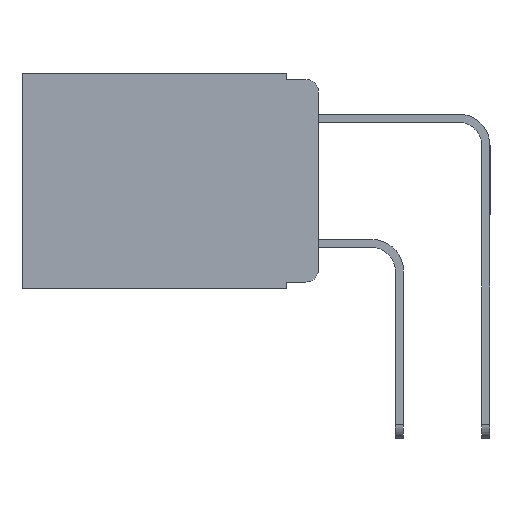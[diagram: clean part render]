
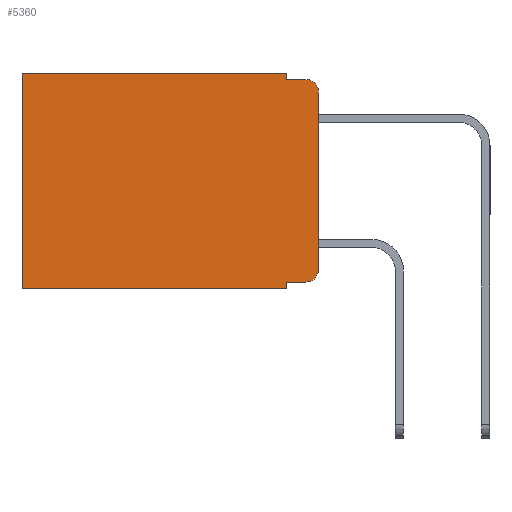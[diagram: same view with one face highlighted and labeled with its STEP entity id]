
A CAD part, left-side view. The second image highlights one B-rep face of the part: STEP entity #5360.
In plain terms, the highlighted planar face has unit normal (-1, 0, 0).
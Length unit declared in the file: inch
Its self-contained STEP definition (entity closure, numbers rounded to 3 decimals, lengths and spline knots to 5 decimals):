
#64 = VERTEX_POINT ( 'NONE', #9106 ) ;
#231 = EDGE_LOOP ( 'NONE', ( #799, #5601, #1090, #2613, #10460, #2832, #511, #421, #3322, #2909 ) ) ;
#248 = EDGE_CURVE ( 'NONE', #4413, #12292, #5980, .T. ) ;
#421 = ORIENTED_EDGE ( 'NONE', *, *, #8925, .F. ) ;
#511 = ORIENTED_EDGE ( 'NONE', *, *, #3131, .F. ) ;
#660 = CARTESIAN_POINT ( 'NONE',  ( 0.298, 0.473, 0. ) ) ;
#770 = CARTESIAN_POINT ( 'NONE',  ( 0.298, 0.051, -0.333 ) ) ;
#799 = ORIENTED_EDGE ( 'NONE', *, *, #2917, .F. ) ;
#839 = EDGE_CURVE ( 'NONE', #64, #4199, #1407, .T. ) ;
#1090 = ORIENTED_EDGE ( 'NONE', *, *, #248, .F. ) ;
#1407 = LINE ( 'NONE', #8912, #4259 ) ;
#1608 = EDGE_CURVE ( 'NONE', #7378, #12292, #6070, .T. ) ;
#1826 = VECTOR ( 'NONE', #3540, 39.37008 ) ;
#1847 = CARTESIAN_POINT ( 'NONE',  ( 0.298, 0.02, -0.313 ) ) ;
#2059 = LINE ( 'NONE', #660, #9380 ) ;
#2218 = DIRECTION ( 'NONE',  ( 0., 0., -1. ) ) ;
#2267 = CIRCLE ( 'NONE', #11400, 0.02 ) ;
#2272 = LINE ( 'NONE', #7502, #11727 ) ;
#2394 = CARTESIAN_POINT ( 'NONE',  ( 0.298, 0.473, -0.343 ) ) ;
#2399 = VECTOR ( 'NONE', #8474, 39.37008 ) ;
#2431 = LINE ( 'NONE', #2488, #1826 ) ;
#2488 = CARTESIAN_POINT ( 'NONE',  ( 0.298, 0., 0. ) ) ;
#2562 = CARTESIAN_POINT ( 'NONE',  ( 0.298, 0.02, -0.333 ) ) ;
#2613 = ORIENTED_EDGE ( 'NONE', *, *, #11981, .F. ) ;
#2786 = VERTEX_POINT ( 'NONE', #2562 ) ;
#2829 = DIRECTION ( 'NONE',  ( 0., 0., -1. ) ) ;
#2832 = ORIENTED_EDGE ( 'NONE', *, *, #10750, .T. ) ;
#2909 = ORIENTED_EDGE ( 'NONE', *, *, #7652, .T. ) ;
#2917 = EDGE_CURVE ( 'NONE', #7378, #9692, #2431, .T. ) ;
#3131 = EDGE_CURVE ( 'NONE', #12172, #10574, #2272, .T. ) ;
#3322 = ORIENTED_EDGE ( 'NONE', *, *, #8294, .T. ) ;
#3540 = DIRECTION ( 'NONE',  ( 0., 0., -1. ) ) ;
#3930 = CARTESIAN_POINT ( 'NONE',  ( 0.298, 0.051, -0.343 ) ) ;
#3992 = CARTESIAN_POINT ( 'NONE',  ( 0.298, 0.473, 0. ) ) ;
#4199 = VERTEX_POINT ( 'NONE', #3992 ) ;
#4259 = VECTOR ( 'NONE', #11810, 39.37008 ) ;
#4413 = VERTEX_POINT ( 'NONE', #5034 ) ;
#5034 = CARTESIAN_POINT ( 'NONE',  ( 0.298, 0.051, -0.01 ) ) ;
#5148 = VECTOR ( 'NONE', #5553, 39.37008 ) ;
#5175 = DIRECTION ( 'NONE',  ( 1., 0., 0. ) ) ;
#5280 = PLANE ( 'NONE',  #8699 ) ;
#5284 = VERTEX_POINT ( 'NONE', #8490 ) ;
#5310 = CARTESIAN_POINT ( 'NONE',  ( 0.298, 0.051, 0. ) ) ;
#5360 = ADVANCED_FACE ( 'NONE', ( #11406 ), #5280, .F. ) ;
#5553 = DIRECTION ( 'NONE',  ( 0., 0., -1. ) ) ;
#5601 = ORIENTED_EDGE ( 'NONE', *, *, #1608, .T. ) ;
#5980 = LINE ( 'NONE', #10342, #9808 ) ;
#6070 = CIRCLE ( 'NONE', #11501, 0.02 ) ;
#6178 = CARTESIAN_POINT ( 'NONE',  ( 0.298, 0., 0. ) ) ;
#7170 = CARTESIAN_POINT ( 'NONE',  ( 0.298, 0., -0.03 ) ) ;
#7378 = VERTEX_POINT ( 'NONE', #7170 ) ;
#7502 = CARTESIAN_POINT ( 'NONE',  ( 0.298, 0., -0.343 ) ) ;
#7509 = LINE ( 'NONE', #770, #2399 ) ;
#7652 = EDGE_CURVE ( 'NONE', #2786, #9692, #2267, .T. ) ;
#7951 = LINE ( 'NONE', #5310, #10117 ) ;
#8294 = EDGE_CURVE ( 'NONE', #5284, #2786, #7509, .T. ) ;
#8474 = DIRECTION ( 'NONE',  ( 0., -1., 0. ) ) ;
#8490 = CARTESIAN_POINT ( 'NONE',  ( 0.298, 0.051, -0.333 ) ) ;
#8573 = DIRECTION ( 'NONE',  ( -1., 0., 0. ) ) ;
#8640 = LINE ( 'NONE', #11189, #5148 ) ;
#8699 = AXIS2_PLACEMENT_3D ( 'NONE', #6178, #5175, #2218 ) ;
#8912 = CARTESIAN_POINT ( 'NONE',  ( 0.298, 0., 0. ) ) ;
#8925 = EDGE_CURVE ( 'NONE', #5284, #12172, #7951, .T. ) ;
#8933 = DIRECTION ( 'NONE',  ( 0., 1., 0. ) ) ;
#8987 = DIRECTION ( 'NONE',  ( 0., -1., 0. ) ) ;
#9106 = CARTESIAN_POINT ( 'NONE',  ( 0.298, 0.051, 0. ) ) ;
#9135 = DIRECTION ( 'NONE',  ( 0., 0., -1. ) ) ;
#9189 = CARTESIAN_POINT ( 'NONE',  ( 0.298, 0.02, -0.03 ) ) ;
#9210 = DIRECTION ( 'NONE',  ( -1., 0., 0. ) ) ;
#9380 = VECTOR ( 'NONE', #10197, 39.37008 ) ;
#9692 = VERTEX_POINT ( 'NONE', #11281 ) ;
#9808 = VECTOR ( 'NONE', #8987, 39.37008 ) ;
#10117 = VECTOR ( 'NONE', #10971, 39.37008 ) ;
#10197 = DIRECTION ( 'NONE',  ( 0., 0., -1. ) ) ;
#10342 = CARTESIAN_POINT ( 'NONE',  ( 0.298, 0.051, -0.01 ) ) ;
#10460 = ORIENTED_EDGE ( 'NONE', *, *, #839, .T. ) ;
#10574 = VERTEX_POINT ( 'NONE', #2394 ) ;
#10750 = EDGE_CURVE ( 'NONE', #4199, #10574, #2059, .T. ) ;
#10971 = DIRECTION ( 'NONE',  ( 0., 0., -1. ) ) ;
#11189 = CARTESIAN_POINT ( 'NONE',  ( 0.298, 0.051, 0. ) ) ;
#11281 = CARTESIAN_POINT ( 'NONE',  ( 0.298, 0., -0.313 ) ) ;
#11400 = AXIS2_PLACEMENT_3D ( 'NONE', #1847, #8573, #2829 ) ;
#11406 = FACE_OUTER_BOUND ( 'NONE', #231, .T. ) ;
#11501 = AXIS2_PLACEMENT_3D ( 'NONE', #9189, #9210, #9135 ) ;
#11665 = CARTESIAN_POINT ( 'NONE',  ( 0.298, 0.02, -0.01 ) ) ;
#11727 = VECTOR ( 'NONE', #8933, 39.37008 ) ;
#11810 = DIRECTION ( 'NONE',  ( 0., 1., 0. ) ) ;
#11981 = EDGE_CURVE ( 'NONE', #64, #4413, #8640, .T. ) ;
#12172 = VERTEX_POINT ( 'NONE', #3930 ) ;
#12292 = VERTEX_POINT ( 'NONE', #11665 ) ;
